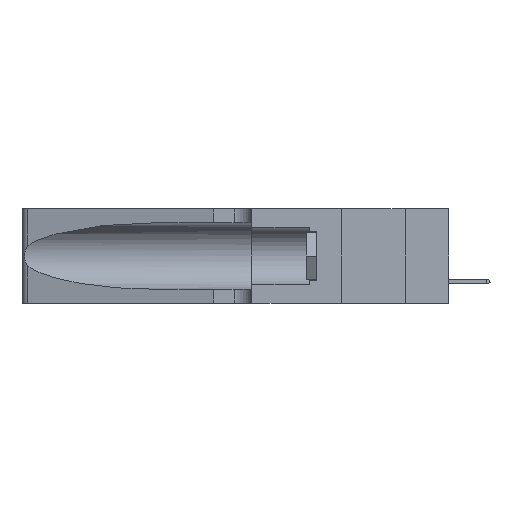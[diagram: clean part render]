
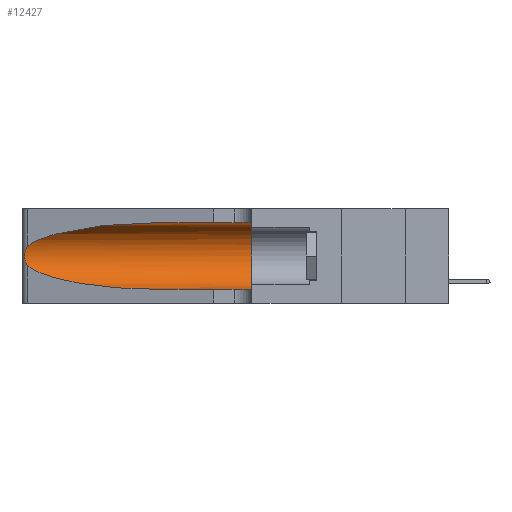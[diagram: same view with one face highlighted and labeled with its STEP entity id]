
A CAD part, left-side view. The second image highlights one B-rep face of the part: STEP entity #12427.
In plain terms, the highlighted cylindrical face has radius 3.308 mm (diameter 6.617 mm), a partial arc.
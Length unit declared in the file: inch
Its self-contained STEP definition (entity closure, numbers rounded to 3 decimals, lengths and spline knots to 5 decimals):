
#48 = CARTESIAN_POINT ( 'NONE',  ( 0.1305, 0.72297, 0.05475 ) ) ;
#253 = CYLINDRICAL_SURFACE ( 'NONE', #9266, 0.13025 ) ;
#683 = CARTESIAN_POINT ( 'NONE',  ( 0.25487, 1.22718, 0.22369 ) ) ;
#1872 = VERTEX_POINT ( 'NONE', #48 ) ;
#2206 = ORIENTED_EDGE ( 'NONE', *, *, #7076, .F. ) ;
#2502 = EDGE_LOOP ( 'NONE', ( #11741, #24200, #23687, #11642, #2206, #27722 ) ) ;
#2950 = CARTESIAN_POINT ( 'NONE',  ( 0.25789, 1.23486, 0.15765 ) ) ;
#3703 = CARTESIAN_POINT ( 'NONE',  ( 0.2373, 1.15595, 0.28018 ) ) ;
#4430 = VERTEX_POINT ( 'NONE', #10865 ) ;
#4670 = CARTESIAN_POINT ( 'NONE',  ( 0.1305, 0.72297, 0.31525 ) ) ;
#4897 = CIRCLE ( 'NONE', #16102, 0.13025 ) ;
#5048 = CARTESIAN_POINT ( 'NONE',  ( 0.26075, 1.23896, 0.178 ) ) ;
#5049 = CARTESIAN_POINT ( 'NONE',  ( 0.1305, 1.61858, 0.05475 ) ) ;
#5906 = VERTEX_POINT ( 'NONE', #23685 ) ;
#7052 = EDGE_CURVE ( 'NONE', #21280, #5906, #22260, .T. ) ;
#7076 = EDGE_CURVE ( 'NONE', #18482, #7195, #4897, .T. ) ;
#7195 = VERTEX_POINT ( 'NONE', #10605 ) ;
#8902 = CARTESIAN_POINT ( 'NONE',  ( 0.1305, 0.35, 0.31525 ) ) ;
#9266 = AXIS2_PLACEMENT_3D ( 'NONE', #11169, #13563, #22179 ) ;
#9337 = CARTESIAN_POINT ( 'NONE',  ( 0.18966, 0.96281, 0.05475 ) ) ;
#9778 = CARTESIAN_POINT ( 'NONE',  ( 0.18966, 0.96281, 0.31525 ) ) ;
#10605 = CARTESIAN_POINT ( 'NONE',  ( 0.1305, 0.35, 0.05475 ) ) ;
#10865 = CARTESIAN_POINT ( 'NONE',  ( 0.25487, 1.22718, 0.14631 ) ) ;
#11169 = CARTESIAN_POINT ( 'NONE',  ( 0.1305, 1.61858, 0.185 ) ) ;
#11445 = EDGE_CURVE ( 'NONE', #4430, #1872, #24002, .T. ) ;
#11616 = CARTESIAN_POINT ( 'NONE',  ( 0.26075, 1.23896, 0.19203 ) ) ;
#11642 = ORIENTED_EDGE ( 'NONE', *, *, #21879, .T. ) ;
#11741 = ORIENTED_EDGE ( 'NONE', *, *, #7052, .T. ) ;
#12177 = VECTOR ( 'NONE', #16218, 39.37008 ) ;
#12306 = VECTOR ( 'NONE', #18342, 39.37008 ) ;
#12427 = ADVANCED_FACE ( 'NONE', ( #23209 ), #253, .F. ) ;
#12934 = EDGE_CURVE ( 'NONE', #5906, #4430, #19443, .T. ) ;
#13563 = DIRECTION ( 'NONE',  ( 0., -1., 0. ) ) ;
#13721 = CARTESIAN_POINT ( 'NONE',  ( 0.25787, 1.23484, 0.2124 ) ) ;
#14406 = EDGE_CURVE ( 'NONE', #21280, #18482, #16449, .T. ) ;
#14488 = CARTESIAN_POINT ( 'NONE',  ( 0.1305, 0.72297, 0.31525 ) ) ;
#15933 = CARTESIAN_POINT ( 'NONE',  ( 0.25639, 1.23184, 0.21858 ) ) ;
#16102 = AXIS2_PLACEMENT_3D ( 'NONE', #24712, #18287, #18198 ) ;
#16218 = DIRECTION ( 'NONE',  ( 0., -1., 0. ) ) ;
#16449 = LINE ( 'NONE', #18059, #12306 ) ;
#18032 = CARTESIAN_POINT ( 'NONE',  ( 0.25487, 1.22718, 0.14631 ) ) ;
#18059 = CARTESIAN_POINT ( 'NONE',  ( 0.1305, 1.61858, 0.31525 ) ) ;
#18198 = DIRECTION ( 'NONE',  ( 0., 0., 1. ) ) ;
#18287 = DIRECTION ( 'NONE',  ( 0., 1., 0. ) ) ;
#18342 = DIRECTION ( 'NONE',  ( 0., -1., 0. ) ) ;
#18482 = VERTEX_POINT ( 'NONE', #8902 ) ;
#19443 = B_SPLINE_CURVE_WITH_KNOTS ( 'NONE', 3,
 ( #683, #20032, #15933, #13721, #26778, #22249, #11616, #5048, #24740, #24548, #2950, #20323, #24440, #18032 ),
 .UNSPECIFIED., .F., .F.,
 ( 4, 2, 2, 2, 2, 2, 4 ),
 ( 0., 0.00027, 0.00053, 0.00107, 0.0016, 0.00187, 0.00214 ),
 .UNSPECIFIED. ) ;
#20032 = CARTESIAN_POINT ( 'NONE',  ( 0.25555, 1.22994, 0.2215 ) ) ;
#20323 = CARTESIAN_POINT ( 'NONE',  ( 0.25639, 1.23186, 0.15144 ) ) ;
#21280 = VERTEX_POINT ( 'NONE', #4670 ) ;
#21879 = EDGE_CURVE ( 'NONE', #1872, #7195, #27600, .T. ) ;
#22179 = DIRECTION ( 'NONE',  ( 0., 0., -1. ) ) ;
#22249 = CARTESIAN_POINT ( 'NONE',  ( 0.26018, 1.23835, 0.19895 ) ) ;
#22260 =( BOUNDED_CURVE ( )  B_SPLINE_CURVE ( 3, ( #14488, #9778, #3703, #27962 ),
 .UNSPECIFIED., .F., .T. ) 
 B_SPLINE_CURVE_WITH_KNOTS ( ( 4, 4 ),
 ( 1.5708, 2.84003 ),
 .UNSPECIFIED. ) 
 CURVE ( )  GEOMETRIC_REPRESENTATION_ITEM ( )  RATIONAL_B_SPLINE_CURVE ( ( 1., 0.87, 0.87, 1. ) ) 
 REPRESENTATION_ITEM ( '' )  );
#23209 = FACE_OUTER_BOUND ( 'NONE', #2502, .T. ) ;
#23685 = CARTESIAN_POINT ( 'NONE',  ( 0.25487, 1.22718, 0.22369 ) ) ;
#23687 = ORIENTED_EDGE ( 'NONE', *, *, #11445, .T. ) ;
#24002 =( BOUNDED_CURVE ( )  B_SPLINE_CURVE ( 3, ( #24561, #24842, #9337, #27074 ),
 .UNSPECIFIED., .F., .F. ) 
 B_SPLINE_CURVE_WITH_KNOTS ( ( 4, 4 ),
 ( 3.44316, 4.71239 ),
 .UNSPECIFIED. ) 
 CURVE ( )  GEOMETRIC_REPRESENTATION_ITEM ( )  RATIONAL_B_SPLINE_CURVE ( ( 1., 0.87, 0.87, 1. ) ) 
 REPRESENTATION_ITEM ( '' )  );
#24200 = ORIENTED_EDGE ( 'NONE', *, *, #12934, .T. ) ;
#24440 = CARTESIAN_POINT ( 'NONE',  ( 0.25555, 1.22993, 0.14849 ) ) ;
#24548 = CARTESIAN_POINT ( 'NONE',  ( 0.25856, 1.23593, 0.16098 ) ) ;
#24561 = CARTESIAN_POINT ( 'NONE',  ( 0.25487, 1.22718, 0.14631 ) ) ;
#24712 = CARTESIAN_POINT ( 'NONE',  ( 0.1305, 0.35, 0.185 ) ) ;
#24740 = CARTESIAN_POINT ( 'NONE',  ( 0.26017, 1.23833, 0.17102 ) ) ;
#24842 = CARTESIAN_POINT ( 'NONE',  ( 0.2373, 1.15595, 0.08982 ) ) ;
#26778 = CARTESIAN_POINT ( 'NONE',  ( 0.25854, 1.2359, 0.20912 ) ) ;
#27074 = CARTESIAN_POINT ( 'NONE',  ( 0.1305, 0.72297, 0.05475 ) ) ;
#27600 = LINE ( 'NONE', #5049, #12177 ) ;
#27722 = ORIENTED_EDGE ( 'NONE', *, *, #14406, .F. ) ;
#27962 = CARTESIAN_POINT ( 'NONE',  ( 0.25487, 1.22718, 0.22369 ) ) ;
